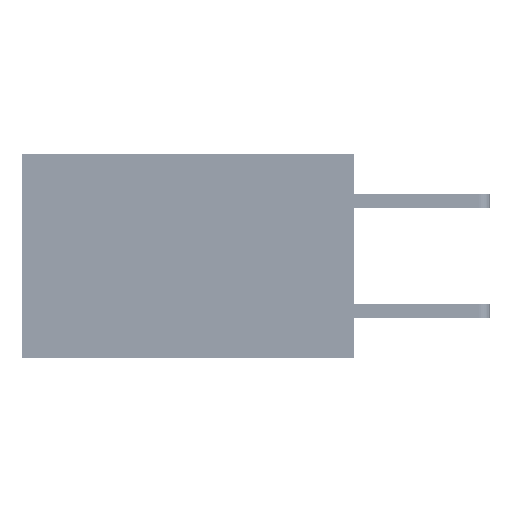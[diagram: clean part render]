
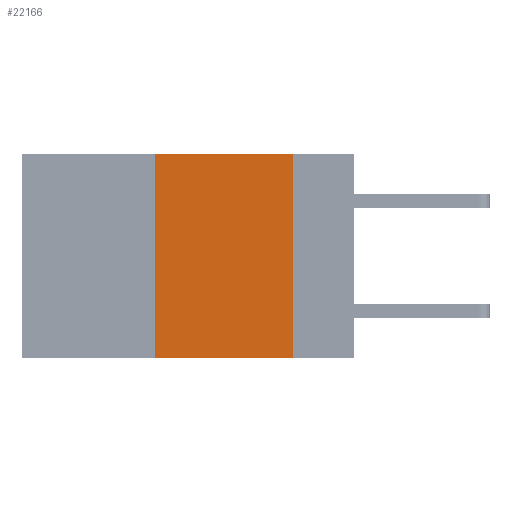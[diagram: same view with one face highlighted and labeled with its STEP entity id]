
A CAD part, left-side view. The second image highlights one B-rep face of the part: STEP entity #22166.
In plain terms, the highlighted planar face has unit normal (-1, 0, 0).
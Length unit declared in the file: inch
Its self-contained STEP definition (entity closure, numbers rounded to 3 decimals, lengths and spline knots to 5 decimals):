
#1110 = CARTESIAN_POINT ( 'NONE',  ( 0., 0.36, 0. ) ) ;
#1187 = CARTESIAN_POINT ( 'NONE',  ( 0., 0.11, 0. ) ) ;
#1697 = VERTEX_POINT ( 'NONE', #21630 ) ;
#2807 = LINE ( 'NONE', #20701, #42472 ) ;
#3906 = DIRECTION ( 'NONE',  ( 0., -1., 0. ) ) ;
#4763 = DIRECTION ( 'NONE',  ( 1., 0., 0. ) ) ;
#6780 = ORIENTED_EDGE ( 'NONE', *, *, #45055, .T. ) ;
#6879 = DIRECTION ( 'NONE',  ( 0., -1., 0. ) ) ;
#8584 = DIRECTION ( 'NONE',  ( 0., 0., -1. ) ) ;
#11087 = ORIENTED_EDGE ( 'NONE', *, *, #11662, .F. ) ;
#11124 = ORIENTED_EDGE ( 'NONE', *, *, #19692, .F. ) ;
#11662 = EDGE_CURVE ( 'NONE', #1697, #11886, #41192, .T. ) ;
#11850 = CARTESIAN_POINT ( 'NONE',  ( 0., 0.36, 0. ) ) ;
#11886 = VERTEX_POINT ( 'NONE', #11850 ) ;
#14234 = VECTOR ( 'NONE', #3906, 39.37008 ) ;
#14814 = VERTEX_POINT ( 'NONE', #43329 ) ;
#15976 = FACE_OUTER_BOUND ( 'NONE', #17368, .T. ) ;
#17368 = EDGE_LOOP ( 'NONE', ( #11124, #36465, #11087, #6780 ) ) ;
#19007 = DIRECTION ( 'NONE',  ( 0., 0., 1. ) ) ;
#19102 = AXIS2_PLACEMENT_3D ( 'NONE', #41727, #4763, #8584 ) ;
#19692 = EDGE_CURVE ( 'NONE', #31409, #14814, #36985, .T. ) ;
#20701 = CARTESIAN_POINT ( 'NONE',  ( 0., 0.6, -0.37 ) ) ;
#21630 = CARTESIAN_POINT ( 'NONE',  ( 0., 0.36, -0.37 ) ) ;
#21800 = CARTESIAN_POINT ( 'NONE',  ( 0., 0.6, 0. ) ) ;
#22166 = ADVANCED_FACE ( 'NONE', ( #15976 ), #31225, .F. ) ;
#25327 = VECTOR ( 'NONE', #19007, 39.37008 ) ;
#28515 = LINE ( 'NONE', #21800, #14234 ) ;
#29545 = VECTOR ( 'NONE', #29599, 39.37008 ) ;
#29599 = DIRECTION ( 'NONE',  ( 0., 0., -1. ) ) ;
#31225 = PLANE ( 'NONE',  #19102 ) ;
#31409 = VERTEX_POINT ( 'NONE', #36164 ) ;
#36164 = CARTESIAN_POINT ( 'NONE',  ( 0., 0.11, 0. ) ) ;
#36465 = ORIENTED_EDGE ( 'NONE', *, *, #42322, .F. ) ;
#36985 = LINE ( 'NONE', #1187, #29545 ) ;
#41192 = LINE ( 'NONE', #1110, #25327 ) ;
#41727 = CARTESIAN_POINT ( 'NONE',  ( 0., 0.6, 0. ) ) ;
#42322 = EDGE_CURVE ( 'NONE', #11886, #31409, #28515, .T. ) ;
#42472 = VECTOR ( 'NONE', #6879, 39.37008 ) ;
#43329 = CARTESIAN_POINT ( 'NONE',  ( 0., 0.11, -0.37 ) ) ;
#45055 = EDGE_CURVE ( 'NONE', #1697, #14814, #2807, .T. ) ;
